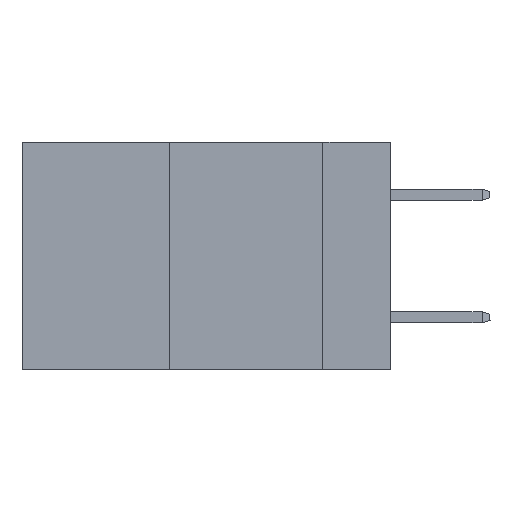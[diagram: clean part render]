
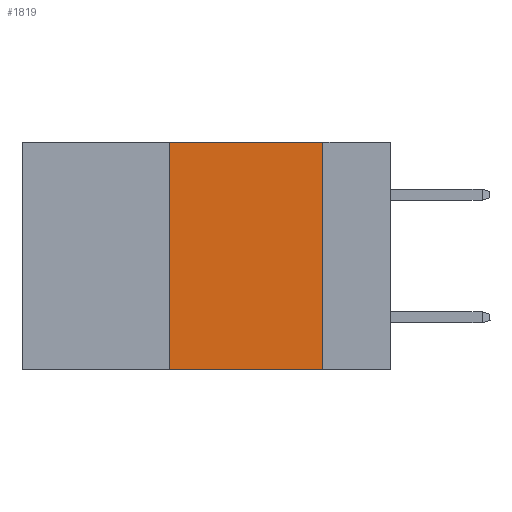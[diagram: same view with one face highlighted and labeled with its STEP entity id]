
A CAD part, left-side view. The second image highlights one B-rep face of the part: STEP entity #1819.
In plain terms, the highlighted planar face has unit normal (-1, 0, 0).
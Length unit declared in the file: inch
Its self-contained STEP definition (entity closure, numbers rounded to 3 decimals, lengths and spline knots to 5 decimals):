
#164 = EDGE_LOOP ( 'NONE', ( #6903, #15637, #5520, #13806 ) ) ;
#911 = EDGE_CURVE ( 'NONE', #9626, #9591, #17213, .T. ) ;
#984 = DIRECTION ( 'NONE',  ( 0., 0., -1. ) ) ;
#1038 = DIRECTION ( 'NONE',  ( 0., 0., -1. ) ) ;
#1634 = VECTOR ( 'NONE', #16319, 39.37008 ) ;
#1819 = ADVANCED_FACE ( 'NONE', ( #2067 ), #10985, .F. ) ;
#1879 = LINE ( 'NONE', #17126, #9229 ) ;
#2067 = FACE_OUTER_BOUND ( 'NONE', #164, .T. ) ;
#2685 = VECTOR ( 'NONE', #5591, 39.37008 ) ;
#3170 = DIRECTION ( 'NONE',  ( 1., 0., 0. ) ) ;
#5520 = ORIENTED_EDGE ( 'NONE', *, *, #14030, .F. ) ;
#5591 = DIRECTION ( 'NONE',  ( 0., -1., 0. ) ) ;
#5787 = LINE ( 'NONE', #12285, #17034 ) ;
#6412 = DIRECTION ( 'NONE',  ( 0., 0., 1. ) ) ;
#6457 = VERTEX_POINT ( 'NONE', #18045 ) ;
#6903 = ORIENTED_EDGE ( 'NONE', *, *, #7334, .F. ) ;
#7334 = EDGE_CURVE ( 'NONE', #9591, #6457, #1879, .T. ) ;
#8020 = VERTEX_POINT ( 'NONE', #18496 ) ;
#8664 = AXIS2_PLACEMENT_3D ( 'NONE', #10826, #3170, #1038 ) ;
#9229 = VECTOR ( 'NONE', #984, 39.37008 ) ;
#9591 = VERTEX_POINT ( 'NONE', #15181 ) ;
#9626 = VERTEX_POINT ( 'NONE', #12360 ) ;
#10528 = LINE ( 'NONE', #15814, #2685 ) ;
#10826 = CARTESIAN_POINT ( 'NONE',  ( 0., 0.6, 0. ) ) ;
#10985 = PLANE ( 'NONE',  #8664 ) ;
#11671 = EDGE_CURVE ( 'NONE', #8020, #6457, #10528, .T. ) ;
#12285 = CARTESIAN_POINT ( 'NONE',  ( 0., 0.36, 0. ) ) ;
#12360 = CARTESIAN_POINT ( 'NONE',  ( 0., 0.36, 0. ) ) ;
#13806 = ORIENTED_EDGE ( 'NONE', *, *, #11671, .T. ) ;
#14030 = EDGE_CURVE ( 'NONE', #8020, #9626, #5787, .T. ) ;
#15181 = CARTESIAN_POINT ( 'NONE',  ( 0., 0.11, 0. ) ) ;
#15637 = ORIENTED_EDGE ( 'NONE', *, *, #911, .F. ) ;
#15814 = CARTESIAN_POINT ( 'NONE',  ( 0., 0.6, -0.37 ) ) ;
#16319 = DIRECTION ( 'NONE',  ( 0., -1., 0. ) ) ;
#17034 = VECTOR ( 'NONE', #6412, 39.37008 ) ;
#17126 = CARTESIAN_POINT ( 'NONE',  ( 0., 0.11, 0. ) ) ;
#17213 = LINE ( 'NONE', #18164, #1634 ) ;
#18045 = CARTESIAN_POINT ( 'NONE',  ( 0., 0.11, -0.37 ) ) ;
#18164 = CARTESIAN_POINT ( 'NONE',  ( 0., 0.6, 0. ) ) ;
#18496 = CARTESIAN_POINT ( 'NONE',  ( 0., 0.36, -0.37 ) ) ;
